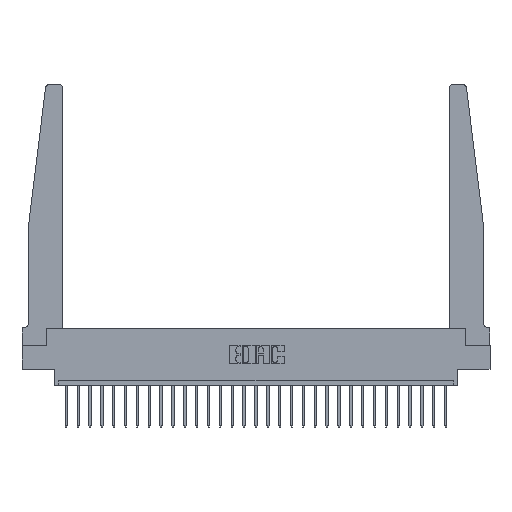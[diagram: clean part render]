
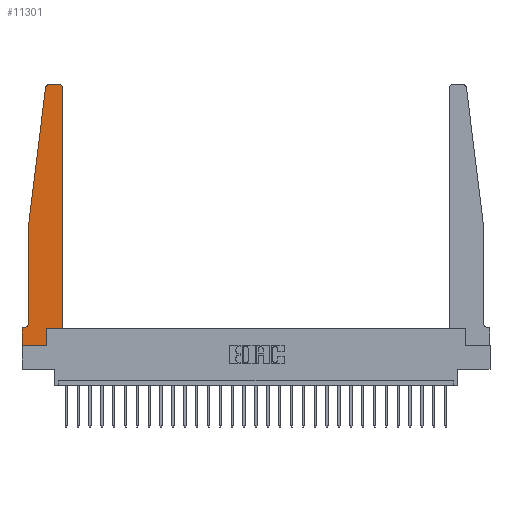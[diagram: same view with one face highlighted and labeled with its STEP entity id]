
A CAD part, top view. The second image highlights one B-rep face of the part: STEP entity #11301.
In plain terms, the highlighted planar face has unit normal (0, 0, 1).
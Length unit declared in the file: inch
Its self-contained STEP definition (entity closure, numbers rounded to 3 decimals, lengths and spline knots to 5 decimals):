
#386 = ORIENTED_EDGE ( 'NONE', *, *, #10260, .T. ) ;
#403 = CARTESIAN_POINT ( 'NONE',  ( 0.395, 2.75, 0.37 ) ) ;
#463 = LINE ( 'NONE', #27013, #6869 ) ;
#473 = EDGE_CURVE ( 'NONE', #7100, #22643, #8513, .T. ) ;
#667 = DIRECTION ( 'NONE',  ( 0., 0., 1. ) ) ;
#858 = DIRECTION ( 'NONE',  ( 1., 0., 0. ) ) ;
#1340 = LINE ( 'NONE', #21999, #24700 ) ;
#1368 = DIRECTION ( 'NONE',  ( 0., 1., 0. ) ) ;
#1571 = LINE ( 'NONE', #17866, #17635 ) ;
#2029 = VERTEX_POINT ( 'NONE', #12727 ) ;
#2807 = ORIENTED_EDGE ( 'NONE', *, *, #21011, .T. ) ;
#4316 = CARTESIAN_POINT ( 'NONE',  ( 0.015, 0.1875, 0.37 ) ) ;
#4317 = EDGE_CURVE ( 'NONE', #23375, #20748, #16700, .T. ) ;
#4798 = DIRECTION ( 'NONE',  ( -1., 0., 0. ) ) ;
#4809 = ORIENTED_EDGE ( 'NONE', *, *, #473, .T. ) ;
#4901 = LINE ( 'NONE', #23772, #5600 ) ;
#4918 = ORIENTED_EDGE ( 'NONE', *, *, #4317, .T. ) ;
#5036 = DIRECTION ( 'NONE',  ( -0.122, -0.992, 0. ) ) ;
#5080 = VECTOR ( 'NONE', #11647, 39.37008 ) ;
#5166 = CARTESIAN_POINT ( 'NONE',  ( 0.425, 0.18, 0.37 ) ) ;
#5363 = CARTESIAN_POINT ( 'NONE',  ( 0.27653, 2.72, 0.37 ) ) ;
#5450 = DIRECTION ( 'NONE',  ( 1., 0., 0. ) ) ;
#5600 = VECTOR ( 'NONE', #5036, 39.37008 ) ;
#6419 = ORIENTED_EDGE ( 'NONE', *, *, #14890, .T. ) ;
#6437 = DIRECTION ( 'NONE',  ( 1., 0., 0. ) ) ;
#6869 = VECTOR ( 'NONE', #14431, 39.37008 ) ;
#6942 = CARTESIAN_POINT ( 'NONE',  ( 0.065, 0.2375, 0.37 ) ) ;
#7100 = VERTEX_POINT ( 'NONE', #21500 ) ;
#7351 = CARTESIAN_POINT ( 'NONE',  ( 0.27653, 2.75, 0.37 ) ) ;
#7606 = LINE ( 'NONE', #5166, #9501 ) ;
#7681 = VERTEX_POINT ( 'NONE', #17898 ) ;
#7828 = VECTOR ( 'NONE', #12623, 39.37008 ) ;
#7875 = DIRECTION ( 'NONE',  ( -1., 0., 0. ) ) ;
#8063 = CIRCLE ( 'NONE', #10691, 0.03 ) ;
#8154 = EDGE_CURVE ( 'NONE', #23511, #10852, #1571, .T. ) ;
#8472 = CARTESIAN_POINT ( 'NONE',  ( 0.395, 2.72, 0.37 ) ) ;
#8513 = LINE ( 'NONE', #19049, #7828 ) ;
#9501 = VECTOR ( 'NONE', #15956, 39.37008 ) ;
#9709 = CARTESIAN_POINT ( 'NONE',  ( 0.2605, 0.18, 0.37 ) ) ;
#10260 = EDGE_CURVE ( 'NONE', #20154, #12550, #15471, .T. ) ;
#10691 = AXIS2_PLACEMENT_3D ( 'NONE', #5363, #21501, #858 ) ;
#10852 = VERTEX_POINT ( 'NONE', #7351 ) ;
#11301 = ADVANCED_FACE ( 'NONE', ( #17210 ), #13649, .T. ) ;
#11612 = CIRCLE ( 'NONE', #25548, 0.03 ) ;
#11647 = DIRECTION ( 'NONE',  ( -1., 0., 0. ) ) ;
#12505 = CARTESIAN_POINT ( 'NONE',  ( 0.065, 1.25, 0.37 ) ) ;
#12550 = VERTEX_POINT ( 'NONE', #4316 ) ;
#12623 = DIRECTION ( 'NONE',  ( 1., 0., 0. ) ) ;
#12643 = ORIENTED_EDGE ( 'NONE', *, *, #17085, .T. ) ;
#12727 = CARTESIAN_POINT ( 'NONE',  ( 0.2605, 0., 0.37 ) ) ;
#13047 = ORIENTED_EDGE ( 'NONE', *, *, #22513, .T. ) ;
#13269 = EDGE_CURVE ( 'NONE', #12550, #23375, #26171, .T. ) ;
#13649 = PLANE ( 'NONE',  #20288 ) ;
#14091 = LINE ( 'NONE', #9709, #24789 ) ;
#14267 = EDGE_CURVE ( 'NONE', #20473, #20154, #463, .T. ) ;
#14431 = DIRECTION ( 'NONE',  ( 0., -1., 0. ) ) ;
#14533 = VERTEX_POINT ( 'NONE', #20811 ) ;
#14650 = CARTESIAN_POINT ( 'NONE',  ( 0., 0., 0.37 ) ) ;
#14890 = EDGE_CURVE ( 'NONE', #2029, #7100, #14091, .T. ) ;
#15233 = ORIENTED_EDGE ( 'NONE', *, *, #13269, .T. ) ;
#15471 = CIRCLE ( 'NONE', #20690, 0.05 ) ;
#15541 = ORIENTED_EDGE ( 'NONE', *, *, #14267, .T. ) ;
#15574 = DIRECTION ( 'NONE',  ( 1., 0., 0. ) ) ;
#15956 = DIRECTION ( 'NONE',  ( 0., 1., 0. ) ) ;
#16054 = EDGE_CURVE ( 'NONE', #22643, #14533, #7606, .T. ) ;
#16143 = CARTESIAN_POINT ( 'NONE',  ( 0., 0.1875, 0.37 ) ) ;
#16305 = CARTESIAN_POINT ( 'NONE',  ( 0.065, 0.1875, 0.37 ) ) ;
#16700 = LINE ( 'NONE', #14650, #23159 ) ;
#17085 = EDGE_CURVE ( 'NONE', #7681, #20473, #4901, .T. ) ;
#17210 = FACE_OUTER_BOUND ( 'NONE', #22871, .T. ) ;
#17635 = VECTOR ( 'NONE', #7875, 39.37008 ) ;
#17866 = CARTESIAN_POINT ( 'NONE',  ( 0.25, 2.75, 0.37 ) ) ;
#17898 = CARTESIAN_POINT ( 'NONE',  ( 0.24675, 2.72367, 0.37 ) ) ;
#18679 = ORIENTED_EDGE ( 'NONE', *, *, #16054, .T. ) ;
#19049 = CARTESIAN_POINT ( 'NONE',  ( 0.425, 0.18, 0.37 ) ) ;
#20154 = VERTEX_POINT ( 'NONE', #6942 ) ;
#20288 = AXIS2_PLACEMENT_3D ( 'NONE', #23643, #667, #15574 ) ;
#20473 = VERTEX_POINT ( 'NONE', #12505 ) ;
#20690 = AXIS2_PLACEMENT_3D ( 'NONE', #21200, #21067, #4798 ) ;
#20748 = VERTEX_POINT ( 'NONE', #22339 ) ;
#20811 = CARTESIAN_POINT ( 'NONE',  ( 0.425, 2.72, 0.37 ) ) ;
#21011 = EDGE_CURVE ( 'NONE', #10852, #7681, #8063, .T. ) ;
#21067 = DIRECTION ( 'NONE',  ( 0., 0., -1. ) ) ;
#21200 = CARTESIAN_POINT ( 'NONE',  ( 0.015, 0.2375, 0.37 ) ) ;
#21202 = DIRECTION ( 'NONE',  ( 0., 0., 1. ) ) ;
#21500 = CARTESIAN_POINT ( 'NONE',  ( 0.2605, 0.18, 0.37 ) ) ;
#21501 = DIRECTION ( 'NONE',  ( 0., 0., 1. ) ) ;
#21807 = ORIENTED_EDGE ( 'NONE', *, *, #8154, .T. ) ;
#21999 = CARTESIAN_POINT ( 'NONE',  ( 0., 0., 0.37 ) ) ;
#22339 = CARTESIAN_POINT ( 'NONE',  ( 0., 0., 0.37 ) ) ;
#22513 = EDGE_CURVE ( 'NONE', #14533, #23511, #11612, .T. ) ;
#22643 = VERTEX_POINT ( 'NONE', #24722 ) ;
#22813 = ORIENTED_EDGE ( 'NONE', *, *, #23800, .T. ) ;
#22871 = EDGE_LOOP ( 'NONE', ( #21807, #2807, #12643, #15541, #386, #15233, #4918, #22813, #6419, #4809, #18679, #13047 ) ) ;
#23159 = VECTOR ( 'NONE', #25595, 39.37008 ) ;
#23375 = VERTEX_POINT ( 'NONE', #16143 ) ;
#23511 = VERTEX_POINT ( 'NONE', #403 ) ;
#23643 = CARTESIAN_POINT ( 'NONE',  ( 0., 0.1875, 0.37 ) ) ;
#23772 = CARTESIAN_POINT ( 'NONE',  ( 0.065, 1.25, 0.37 ) ) ;
#23800 = EDGE_CURVE ( 'NONE', #20748, #2029, #1340, .T. ) ;
#24700 = VECTOR ( 'NONE', #5450, 39.37008 ) ;
#24722 = CARTESIAN_POINT ( 'NONE',  ( 0.425, 0.18, 0.37 ) ) ;
#24789 = VECTOR ( 'NONE', #1368, 39.37008 ) ;
#25548 = AXIS2_PLACEMENT_3D ( 'NONE', #8472, #21202, #6437 ) ;
#25595 = DIRECTION ( 'NONE',  ( 0., -1., 0. ) ) ;
#26171 = LINE ( 'NONE', #16305, #5080 ) ;
#27013 = CARTESIAN_POINT ( 'NONE',  ( 0.065, 1.25, 0.37 ) ) ;
